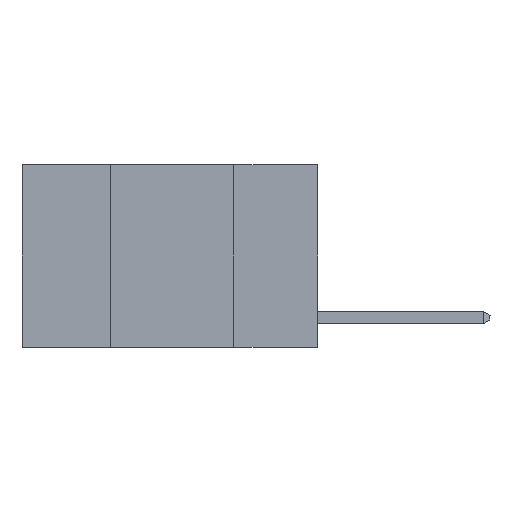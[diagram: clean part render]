
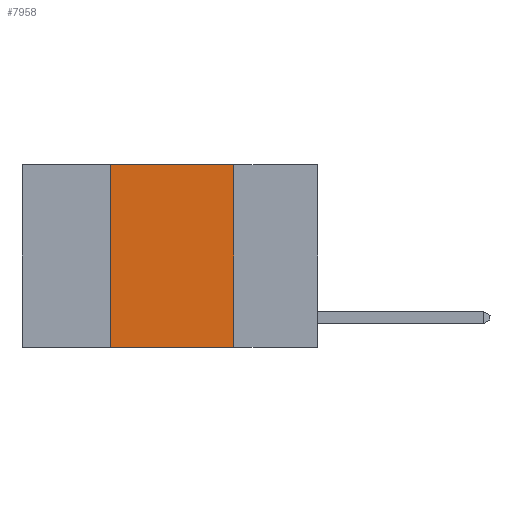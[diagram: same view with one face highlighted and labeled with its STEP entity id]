
A CAD part, left-side view. The second image highlights one B-rep face of the part: STEP entity #7958.
In plain terms, the highlighted planar face has unit normal (-1, 0, 0).
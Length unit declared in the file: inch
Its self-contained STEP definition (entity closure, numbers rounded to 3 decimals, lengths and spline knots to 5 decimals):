
#373 = CARTESIAN_POINT ( 'NONE',  ( 0., 0.6, -0.37 ) ) ;
#498 = VECTOR ( 'NONE', #4496, 39.37008 ) ;
#579 = EDGE_CURVE ( 'NONE', #7090, #2191, #4754, .T. ) ;
#1670 = CARTESIAN_POINT ( 'NONE',  ( 0., 0.6, 0. ) ) ;
#1855 = DIRECTION ( 'NONE',  ( 0., 0., -1. ) ) ;
#1924 = EDGE_CURVE ( 'NONE', #2191, #9047, #4704, .T. ) ;
#1956 = CARTESIAN_POINT ( 'NONE',  ( 0., 0.17, 0. ) ) ;
#1984 = CARTESIAN_POINT ( 'NONE',  ( 0., 0.42, 0. ) ) ;
#2090 = EDGE_LOOP ( 'NONE', ( #3731, #2613, #8468, #8005 ) ) ;
#2191 = VERTEX_POINT ( 'NONE', #1984 ) ;
#2613 = ORIENTED_EDGE ( 'NONE', *, *, #1924, .F. ) ;
#3179 = CARTESIAN_POINT ( 'NONE',  ( 0., 0.42, 0. ) ) ;
#3680 = LINE ( 'NONE', #9900, #498 ) ;
#3731 = ORIENTED_EDGE ( 'NONE', *, *, #8786, .F. ) ;
#4242 = CARTESIAN_POINT ( 'NONE',  ( 0., 0.17, -0.37 ) ) ;
#4339 = VECTOR ( 'NONE', #8336, 39.37008 ) ;
#4458 = DIRECTION ( 'NONE',  ( 0., -1., 0. ) ) ;
#4496 = DIRECTION ( 'NONE',  ( 0., 0., -1. ) ) ;
#4704 = LINE ( 'NONE', #1670, #5422 ) ;
#4754 = LINE ( 'NONE', #3179, #11408 ) ;
#5062 = DIRECTION ( 'NONE',  ( 0., 0., 1. ) ) ;
#5422 = VECTOR ( 'NONE', #4458, 39.37008 ) ;
#6645 = LINE ( 'NONE', #373, #4339 ) ;
#7090 = VERTEX_POINT ( 'NONE', #7313 ) ;
#7219 = PLANE ( 'NONE',  #7900 ) ;
#7303 = EDGE_CURVE ( 'NONE', #7090, #7590, #6645, .T. ) ;
#7313 = CARTESIAN_POINT ( 'NONE',  ( 0., 0.42, -0.37 ) ) ;
#7590 = VERTEX_POINT ( 'NONE', #4242 ) ;
#7615 = FACE_OUTER_BOUND ( 'NONE', #2090, .T. ) ;
#7900 = AXIS2_PLACEMENT_3D ( 'NONE', #8878, #8220, #1855 ) ;
#7958 = ADVANCED_FACE ( 'NONE', ( #7615 ), #7219, .F. ) ;
#8005 = ORIENTED_EDGE ( 'NONE', *, *, #7303, .T. ) ;
#8220 = DIRECTION ( 'NONE',  ( 1., 0., 0. ) ) ;
#8336 = DIRECTION ( 'NONE',  ( 0., -1., 0. ) ) ;
#8468 = ORIENTED_EDGE ( 'NONE', *, *, #579, .F. ) ;
#8786 = EDGE_CURVE ( 'NONE', #9047, #7590, #3680, .T. ) ;
#8878 = CARTESIAN_POINT ( 'NONE',  ( 0., 0.6, 0. ) ) ;
#9047 = VERTEX_POINT ( 'NONE', #1956 ) ;
#9900 = CARTESIAN_POINT ( 'NONE',  ( 0., 0.17, 0. ) ) ;
#11408 = VECTOR ( 'NONE', #5062, 39.37008 ) ;
